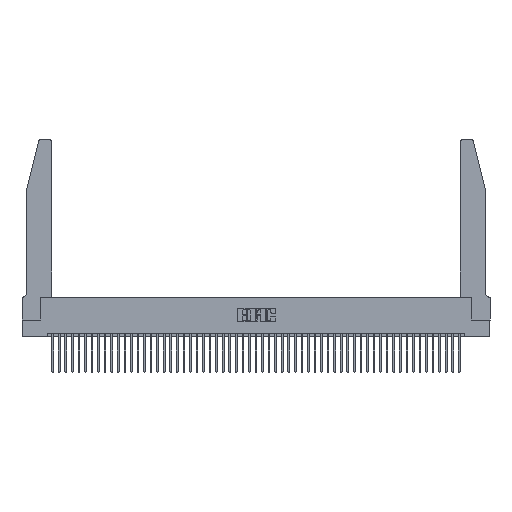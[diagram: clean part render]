
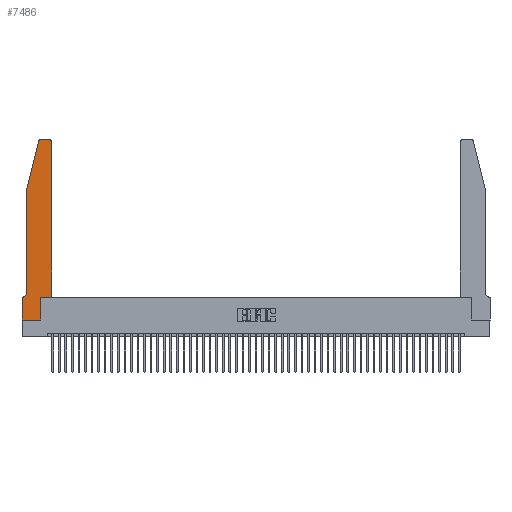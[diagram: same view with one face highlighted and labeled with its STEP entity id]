
A CAD part, top view. The second image highlights one B-rep face of the part: STEP entity #7486.
In plain terms, the highlighted planar face has unit normal (0, 0, 1).
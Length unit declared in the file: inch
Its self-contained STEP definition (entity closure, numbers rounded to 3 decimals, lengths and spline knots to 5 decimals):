
#431 = EDGE_CURVE ( 'NONE', #35367, #9760, #17806, .T. ) ;
#613 = ORIENTED_EDGE ( 'NONE', *, *, #431, .T. ) ;
#671 = EDGE_CURVE ( 'NONE', #45657, #7878, #41344, .T. ) ;
#1345 = LINE ( 'NONE', #45399, #29267 ) ;
#3273 = EDGE_CURVE ( 'NONE', #29829, #35367, #16860, .T. ) ;
#3872 = CARTESIAN_POINT ( 'NONE',  ( 0.4505, 0.35, 0.37 ) ) ;
#4806 = LINE ( 'NONE', #30564, #23374 ) ;
#5410 = EDGE_LOOP ( 'NONE', ( #31438, #40963, #613, #46143, #41574, #12114, #9392, #6717, #35068, #17539, #37433, #45960 ) ) ;
#5556 = DIRECTION ( 'NONE',  ( -1., 0., 0. ) ) ;
#5646 = CARTESIAN_POINT ( 'NONE',  ( 0.0755, 0.42, 0.37 ) ) ;
#6203 = CARTESIAN_POINT ( 'NONE',  ( 0.0755, 2., 0.37 ) ) ;
#6693 = EDGE_CURVE ( 'NONE', #6741, #25845, #23249, .T. ) ;
#6717 = ORIENTED_EDGE ( 'NONE', *, *, #6693, .T. ) ;
#6741 = VERTEX_POINT ( 'NONE', #49063 ) ;
#7486 = ADVANCED_FACE ( 'NONE', ( #19418 ), #43658, .T. ) ;
#7878 = VERTEX_POINT ( 'NONE', #13458 ) ;
#8157 = CARTESIAN_POINT ( 'NONE',  ( 0., 0.35, 0.37 ) ) ;
#9392 = ORIENTED_EDGE ( 'NONE', *, *, #25875, .T. ) ;
#9760 = VERTEX_POINT ( 'NONE', #11988 ) ;
#11047 = CARTESIAN_POINT ( 'NONE',  ( 0.284, 2.72, 0.37 ) ) ;
#11988 = CARTESIAN_POINT ( 'NONE',  ( 0.0755, 2., 0.37 ) ) ;
#12114 = ORIENTED_EDGE ( 'NONE', *, *, #13427, .T. ) ;
#12570 = CIRCLE ( 'NONE', #49219, 0.03 ) ;
#12595 = EDGE_CURVE ( 'NONE', #25845, #45657, #1345, .T. ) ;
#13044 = VECTOR ( 'NONE', #43056, 39.37008 ) ;
#13427 = EDGE_CURVE ( 'NONE', #42847, #43987, #20428, .T. ) ;
#13458 = CARTESIAN_POINT ( 'NONE',  ( 0.4505, 0.35, 0.37 ) ) ;
#13584 = EDGE_CURVE ( 'NONE', #7878, #16348, #19824, .T. ) ;
#13832 = DIRECTION ( 'NONE',  ( 0., 1., 0. ) ) ;
#14126 = CARTESIAN_POINT ( 'NONE',  ( 0., 0., 0.37 ) ) ;
#14427 = DIRECTION ( 'NONE',  ( -1., 0., 0. ) ) ;
#14714 = VECTOR ( 'NONE', #32583, 39.37008 ) ;
#14805 = DIRECTION ( 'NONE',  ( 1., 0., 0. ) ) ;
#15168 = VECTOR ( 'NONE', #41387, 39.37008 ) ;
#16263 = CARTESIAN_POINT ( 'NONE',  ( 0., 0.35, 0.37 ) ) ;
#16348 = VERTEX_POINT ( 'NONE', #29147 ) ;
#16860 = CIRCLE ( 'NONE', #18718, 0.03 ) ;
#17539 = ORIENTED_EDGE ( 'NONE', *, *, #671, .T. ) ;
#17700 = VECTOR ( 'NONE', #41398, 39.37008 ) ;
#17806 = LINE ( 'NONE', #28066, #14714 ) ;
#18718 = AXIS2_PLACEMENT_3D ( 'NONE', #11047, #42771, #22999 ) ;
#19418 = FACE_OUTER_BOUND ( 'NONE', #5410, .T. ) ;
#19824 = LINE ( 'NONE', #3872, #34122 ) ;
#20428 = LINE ( 'NONE', #46375, #13044 ) ;
#20787 = EDGE_CURVE ( 'NONE', #22538, #29829, #4806, .T. ) ;
#21991 = LINE ( 'NONE', #6203, #15168 ) ;
#22078 = CARTESIAN_POINT ( 'NONE',  ( 0.284, 2.75, 0.37 ) ) ;
#22538 = VERTEX_POINT ( 'NONE', #23608 ) ;
#22999 = DIRECTION ( 'NONE',  ( 1., 0., 0. ) ) ;
#23249 = LINE ( 'NONE', #40368, #17700 ) ;
#23374 = VECTOR ( 'NONE', #14427, 39.37008 ) ;
#23608 = CARTESIAN_POINT ( 'NONE',  ( 0.4205, 2.75, 0.37 ) ) ;
#23715 = DIRECTION ( 'NONE',  ( 1., 0., 0. ) ) ;
#23788 = DIRECTION ( 'NONE',  ( 0., 1., 0. ) ) ;
#24166 = LINE ( 'NONE', #14126, #45271 ) ;
#24186 = EDGE_CURVE ( 'NONE', #16348, #22538, #12570, .T. ) ;
#25213 = VECTOR ( 'NONE', #41585, 39.37008 ) ;
#25845 = VERTEX_POINT ( 'NONE', #26083 ) ;
#25875 = EDGE_CURVE ( 'NONE', #43987, #6741, #24166, .T. ) ;
#26083 = CARTESIAN_POINT ( 'NONE',  ( 0.2865, 0., 0.37 ) ) ;
#26714 = CARTESIAN_POINT ( 'NONE',  ( 0.25487, 2.72718, 0.37 ) ) ;
#26931 = DIRECTION ( 'NONE',  ( 0., 0., 1. ) ) ;
#27455 = AXIS2_PLACEMENT_3D ( 'NONE', #16263, #43474, #23715 ) ;
#28066 = CARTESIAN_POINT ( 'NONE',  ( 0.0755, 2., 0.37 ) ) ;
#29147 = CARTESIAN_POINT ( 'NONE',  ( 0.4505, 2.72, 0.37 ) ) ;
#29267 = VECTOR ( 'NONE', #13832, 39.37008 ) ;
#29829 = VERTEX_POINT ( 'NONE', #22078 ) ;
#29924 = AXIS2_PLACEMENT_3D ( 'NONE', #45240, #37940, #5556 ) ;
#30564 = CARTESIAN_POINT ( 'NONE',  ( 0.2605, 2.75, 0.37 ) ) ;
#31438 = ORIENTED_EDGE ( 'NONE', *, *, #20787, .T. ) ;
#32583 = DIRECTION ( 'NONE',  ( -0.239, -0.971, 0. ) ) ;
#33381 = DIRECTION ( 'NONE',  ( 0., -1., 0. ) ) ;
#34122 = VECTOR ( 'NONE', #23788, 39.37008 ) ;
#35068 = ORIENTED_EDGE ( 'NONE', *, *, #12595, .T. ) ;
#35367 = VERTEX_POINT ( 'NONE', #26714 ) ;
#35638 = CIRCLE ( 'NONE', #29924, 0.07 ) ;
#37433 = ORIENTED_EDGE ( 'NONE', *, *, #13584, .T. ) ;
#37587 = CARTESIAN_POINT ( 'NONE',  ( 0.4505, 0.35, 0.37 ) ) ;
#37940 = DIRECTION ( 'NONE',  ( 0., 0., -1. ) ) ;
#40368 = CARTESIAN_POINT ( 'NONE',  ( 0., 0., 0.37 ) ) ;
#40963 = ORIENTED_EDGE ( 'NONE', *, *, #3273, .T. ) ;
#41344 = LINE ( 'NONE', #37587, #25213 ) ;
#41387 = DIRECTION ( 'NONE',  ( 0., -1., 0. ) ) ;
#41398 = DIRECTION ( 'NONE',  ( 1., 0., 0. ) ) ;
#41574 = ORIENTED_EDGE ( 'NONE', *, *, #46780, .T. ) ;
#41585 = DIRECTION ( 'NONE',  ( 1., 0., 0. ) ) ;
#42365 = CARTESIAN_POINT ( 'NONE',  ( 0.4205, 2.72, 0.37 ) ) ;
#42771 = DIRECTION ( 'NONE',  ( 0., 0., 1. ) ) ;
#42847 = VERTEX_POINT ( 'NONE', #44997 ) ;
#42909 = CARTESIAN_POINT ( 'NONE',  ( 0.2865, 0.35, 0.37 ) ) ;
#43056 = DIRECTION ( 'NONE',  ( -1., 0., 0. ) ) ;
#43474 = DIRECTION ( 'NONE',  ( 0., 0., 1. ) ) ;
#43658 = PLANE ( 'NONE',  #27455 ) ;
#43987 = VERTEX_POINT ( 'NONE', #8157 ) ;
#44802 = VERTEX_POINT ( 'NONE', #5646 ) ;
#44997 = CARTESIAN_POINT ( 'NONE',  ( 0.0055, 0.35, 0.37 ) ) ;
#45240 = CARTESIAN_POINT ( 'NONE',  ( 0.0055, 0.42, 0.37 ) ) ;
#45271 = VECTOR ( 'NONE', #33381, 39.37008 ) ;
#45399 = CARTESIAN_POINT ( 'NONE',  ( 0.2865, 0.35, 0.37 ) ) ;
#45657 = VERTEX_POINT ( 'NONE', #42909 ) ;
#45960 = ORIENTED_EDGE ( 'NONE', *, *, #24186, .T. ) ;
#46143 = ORIENTED_EDGE ( 'NONE', *, *, #47292, .T. ) ;
#46375 = CARTESIAN_POINT ( 'NONE',  ( 0.0755, 0.35, 0.37 ) ) ;
#46780 = EDGE_CURVE ( 'NONE', #44802, #42847, #35638, .T. ) ;
#47292 = EDGE_CURVE ( 'NONE', #9760, #44802, #21991, .T. ) ;
#49063 = CARTESIAN_POINT ( 'NONE',  ( 0., 0., 0.37 ) ) ;
#49219 = AXIS2_PLACEMENT_3D ( 'NONE', #42365, #26931, #14805 ) ;
